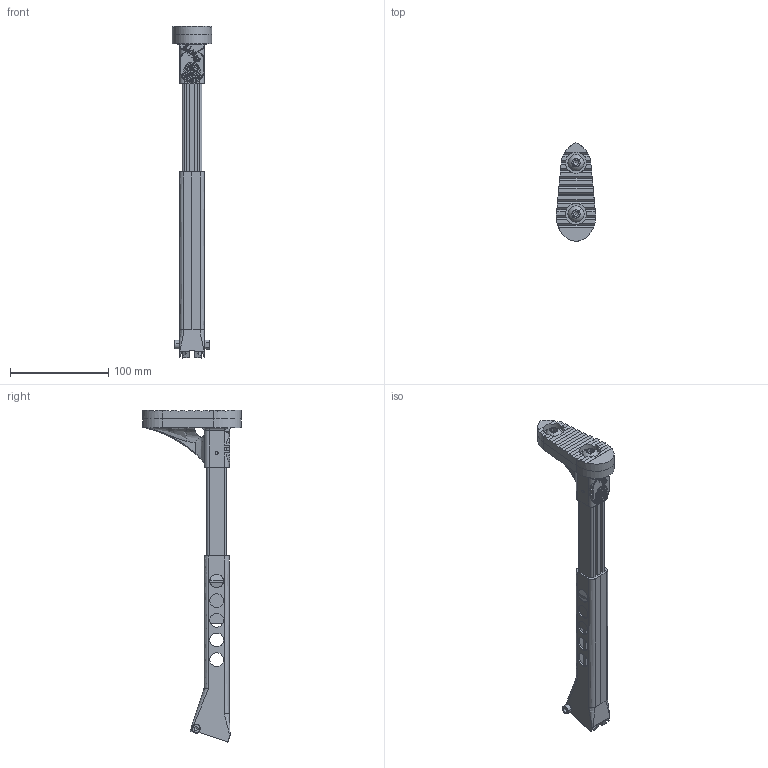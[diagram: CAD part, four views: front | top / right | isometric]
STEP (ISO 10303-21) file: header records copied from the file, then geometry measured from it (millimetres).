
FILE_DESCRIPTION (( 'STEP AP203' ), '1' );
FILE_NAME ('E43x Stock Assembly.STEP', '2020-12-17T02:27:20', ( '' ), ( '' ), 'SwSTEP 2.0', 'SolidWorks 2016', '' );
FILE_SCHEMA (( 'CONFIG_CONTROL_DESIGN' ));
Products named in the file (10): hex nut gradec_bsi_BS EN 24034 - M5 - N; 93R_style_stocktube_Thin Walled; socket head cap screw_bsi_BS EN ISO 4762 M5 x 30 - 22N; parallel pin unhardened_bsi_BS EN ISO 2338 - 3 m6 x 26 - St; 93R_style_stockbar; 93R_style_butplate_Bolted buttpad; 93R_stock_button_mod2; socket button head cap screw_ai_SBHCSCREW 0.375-16x0.5-HX-N; E43x Stock Assembly; 93R_stock_buttpad
Assembly tree (11 placements, depth 2):
  E43x Stock Assembly
    93R_style_stocktube_Thin Walled
    93R_style_stockbar
    93R_style_butplate_Bolted buttpad
    parallel pin unhardened_bsi_BS EN ISO 2338 - 3 m6 x 26 - St
    socket head cap screw_bsi_BS EN ISO 4762 M5 x 30 - 22N
    hex nut gradec_bsi_BS EN 24034 - M5 - N
    93R_stock_button_mod2  x2
    93R_stock_buttpad
    socket button head cap screw_ai_SBHCSCREW 0.375-16x0.5-HX-N  x2
Bounding box: 39.99 x 99.99 x 337.7 mm (x, y, z)
Volume: 197918.4 mm3; surface area: 87933.8 mm2
Topology: 11 solids, 11 shells, 1879 faces, 5344 edges, 3522 vertices
Faces by surface type: plane 1261, cylinder 520, bspline 42, cone 38, torus 14, sphere 4
Entity records: 66533 total; most frequent: CARTESIAN_POINT 17255, ORIENTED_EDGE 10484, DIRECTION 9589, EDGE_CURVE 5242, VECTOR 3963, LINE 3963, VERTEX_POINT 3464, AXIS2_PLACEMENT_3D 2813
